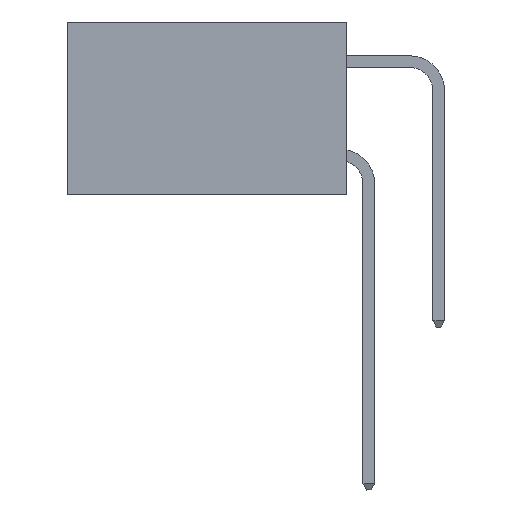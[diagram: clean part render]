
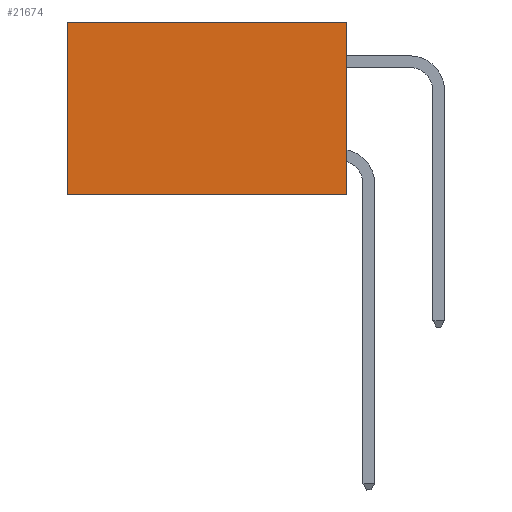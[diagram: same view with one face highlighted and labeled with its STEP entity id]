
A CAD part, left-side view. The second image highlights one B-rep face of the part: STEP entity #21674.
In plain terms, the highlighted planar face has unit normal (-1, 0, 0).
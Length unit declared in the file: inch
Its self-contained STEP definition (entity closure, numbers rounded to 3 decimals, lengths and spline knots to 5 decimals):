
#2108 = DIRECTION ( 'NONE',  ( 0., 1., 0. ) ) ;
#2546 = VECTOR ( 'NONE', #26957, 39.37008 ) ;
#3844 = EDGE_CURVE ( 'NONE', #28843, #21220, #12973, .T. ) ;
#3935 = EDGE_CURVE ( 'NONE', #8412, #17219, #30519, .T. ) ;
#3983 = LINE ( 'NONE', #6702, #14798 ) ;
#6483 = CARTESIAN_POINT ( 'NONE',  ( 0.2875, 0.6, 0. ) ) ;
#6702 = CARTESIAN_POINT ( 'NONE',  ( 0.2875, 0., 0. ) ) ;
#7252 = EDGE_LOOP ( 'NONE', ( #23715, #13561, #29453, #23822 ) ) ;
#7286 = CARTESIAN_POINT ( 'NONE',  ( 0.2875, 0., -0.37 ) ) ;
#7661 = EDGE_CURVE ( 'NONE', #8412, #28843, #3983, .T. ) ;
#7878 = CARTESIAN_POINT ( 'NONE',  ( 0.2875, 0.6, 0. ) ) ;
#8114 = CARTESIAN_POINT ( 'NONE',  ( 0.2875, 0.6, -0.37 ) ) ;
#8412 = VERTEX_POINT ( 'NONE', #14702 ) ;
#9055 = VECTOR ( 'NONE', #2108, 39.37008 ) ;
#9751 = PLANE ( 'NONE',  #27321 ) ;
#12179 = VECTOR ( 'NONE', #22075, 39.37008 ) ;
#12973 = LINE ( 'NONE', #6483, #2546 ) ;
#13561 = ORIENTED_EDGE ( 'NONE', *, *, #14856, .F. ) ;
#14702 = CARTESIAN_POINT ( 'NONE',  ( 0.2875, 0., 0. ) ) ;
#14755 = DIRECTION ( 'NONE',  ( 0., 1., 0. ) ) ;
#14798 = VECTOR ( 'NONE', #14755, 39.37008 ) ;
#14856 = EDGE_CURVE ( 'NONE', #17219, #21220, #24977, .T. ) ;
#15142 = DIRECTION ( 'NONE',  ( 1., 0., 0. ) ) ;
#17219 = VERTEX_POINT ( 'NONE', #22672 ) ;
#17366 = DIRECTION ( 'NONE',  ( 0., 0., -1. ) ) ;
#21220 = VERTEX_POINT ( 'NONE', #8114 ) ;
#21674 = ADVANCED_FACE ( 'NONE', ( #32084 ), #9751, .F. ) ;
#22075 = DIRECTION ( 'NONE',  ( 0., 0., -1. ) ) ;
#22672 = CARTESIAN_POINT ( 'NONE',  ( 0.2875, 0., -0.37 ) ) ;
#22783 = CARTESIAN_POINT ( 'NONE',  ( 0.2875, 0., 0. ) ) ;
#23715 = ORIENTED_EDGE ( 'NONE', *, *, #3844, .T. ) ;
#23822 = ORIENTED_EDGE ( 'NONE', *, *, #7661, .T. ) ;
#24977 = LINE ( 'NONE', #7286, #9055 ) ;
#26957 = DIRECTION ( 'NONE',  ( 0., 0., -1. ) ) ;
#27321 = AXIS2_PLACEMENT_3D ( 'NONE', #22783, #15142, #17366 ) ;
#27502 = CARTESIAN_POINT ( 'NONE',  ( 0.2875, 0., 0. ) ) ;
#28843 = VERTEX_POINT ( 'NONE', #7878 ) ;
#29453 = ORIENTED_EDGE ( 'NONE', *, *, #3935, .F. ) ;
#30519 = LINE ( 'NONE', #27502, #12179 ) ;
#32084 = FACE_OUTER_BOUND ( 'NONE', #7252, .T. ) ;
